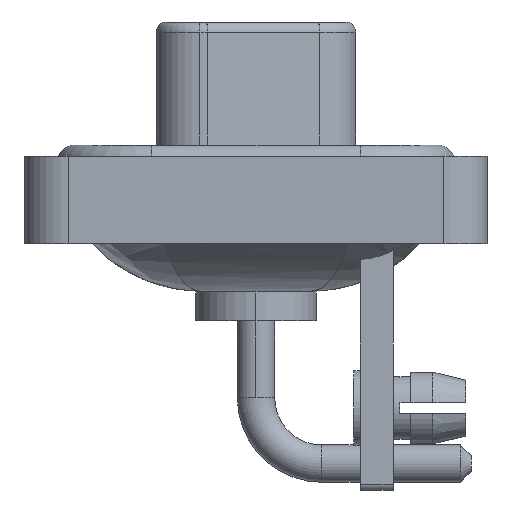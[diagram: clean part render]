
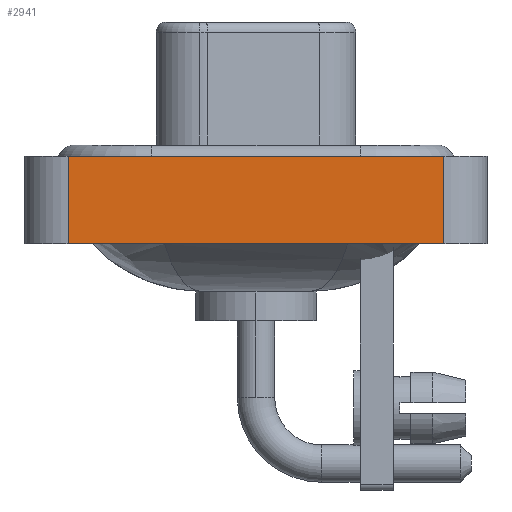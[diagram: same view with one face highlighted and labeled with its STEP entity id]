
A CAD part, left-side view. The second image highlights one B-rep face of the part: STEP entity #2941.
In plain terms, the highlighted planar face has unit normal (-1, 0, 0).
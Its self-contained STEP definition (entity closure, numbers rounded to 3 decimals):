
#1778 = VERTEX_POINT ( 'NONE', #6923 ) ;
#2047 = ORIENTED_EDGE ( 'NONE', *, *, #4397, .T. ) ;
#2401 = LINE ( 'NONE', #16352, #14010 ) ;
#2553 = EDGE_LOOP ( 'NONE', ( #6061, #19122, #11836, #2047 ) ) ;
#2941 = ADVANCED_FACE ( 'NONE', ( #5930 ), #7691, .T. ) ;
#3700 = CARTESIAN_POINT ( 'NONE',  ( -7.35, 8.55, -3.6 ) ) ;
#4263 = CARTESIAN_POINT ( 'NONE',  ( -7.35, -8.55, -3.6 ) ) ;
#4397 = EDGE_CURVE ( 'NONE', #18275, #19544, #17493, .T. ) ;
#5930 = FACE_OUTER_BOUND ( 'NONE', #2553, .T. ) ;
#6061 = ORIENTED_EDGE ( 'NONE', *, *, #9239, .T. ) ;
#6923 = CARTESIAN_POINT ( 'NONE',  ( -7.35, -8.55, 0.4 ) ) ;
#7592 = DIRECTION ( 'NONE',  ( 0., 0., 1. ) ) ;
#7596 = CARTESIAN_POINT ( 'NONE',  ( -7.35, 8.55, 0.4 ) ) ;
#7691 = PLANE ( 'NONE',  #14527 ) ;
#8345 = DIRECTION ( 'NONE',  ( 0., -1., 0. ) ) ;
#8977 = EDGE_CURVE ( 'NONE', #9007, #1778, #18129, .T. ) ;
#9007 = VERTEX_POINT ( 'NONE', #7596 ) ;
#9227 = DIRECTION ( 'NONE',  ( 0., 0., 1. ) ) ;
#9239 = EDGE_CURVE ( 'NONE', #19544, #1778, #2401, .T. ) ;
#9773 = DIRECTION ( 'NONE',  ( 0., -1., 0. ) ) ;
#10004 = VECTOR ( 'NONE', #9227, 1000. ) ;
#11836 = ORIENTED_EDGE ( 'NONE', *, *, #16798, .F. ) ;
#12231 = VECTOR ( 'NONE', #9773, 1000. ) ;
#14010 = VECTOR ( 'NONE', #18111, 1000. ) ;
#14527 = AXIS2_PLACEMENT_3D ( 'NONE', #4263, #15241, #7592 ) ;
#15241 = DIRECTION ( 'NONE',  ( -1., 0., 0. ) ) ;
#16056 = CARTESIAN_POINT ( 'NONE',  ( -7.35, -8.55, -3.6 ) ) ;
#16185 = CARTESIAN_POINT ( 'NONE',  ( -7.35, -8.55, -3.6 ) ) ;
#16352 = CARTESIAN_POINT ( 'NONE',  ( -7.35, -8.55, -3.6 ) ) ;
#16671 = CARTESIAN_POINT ( 'NONE',  ( -7.35, -8.55, 0.4 ) ) ;
#16798 = EDGE_CURVE ( 'NONE', #18275, #9007, #16829, .T. ) ;
#16829 = LINE ( 'NONE', #20040, #10004 ) ;
#17493 = LINE ( 'NONE', #16056, #12231 ) ;
#18111 = DIRECTION ( 'NONE',  ( 0., 0., 1. ) ) ;
#18129 = LINE ( 'NONE', #16671, #18931 ) ;
#18275 = VERTEX_POINT ( 'NONE', #3700 ) ;
#18931 = VECTOR ( 'NONE', #8345, 1000. ) ;
#19122 = ORIENTED_EDGE ( 'NONE', *, *, #8977, .F. ) ;
#19544 = VERTEX_POINT ( 'NONE', #16185 ) ;
#20040 = CARTESIAN_POINT ( 'NONE',  ( -7.35, 8.55, -3.6 ) ) ;
